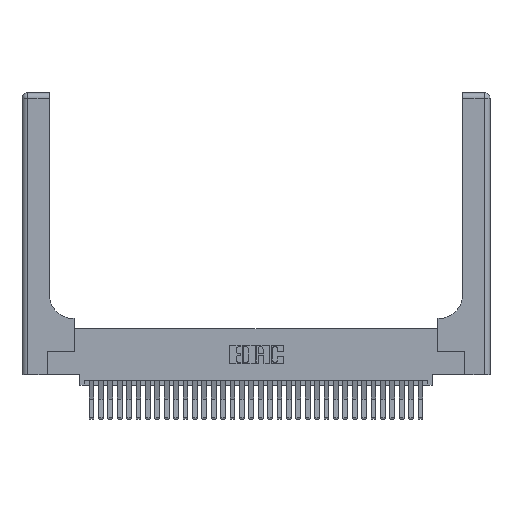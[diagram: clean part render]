
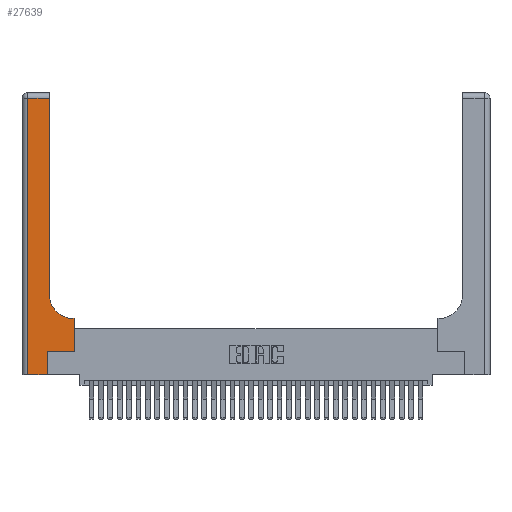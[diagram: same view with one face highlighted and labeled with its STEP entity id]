
A CAD part, top view. The second image highlights one B-rep face of the part: STEP entity #27639.
In plain terms, the highlighted planar face has unit normal (0, 0, 1).
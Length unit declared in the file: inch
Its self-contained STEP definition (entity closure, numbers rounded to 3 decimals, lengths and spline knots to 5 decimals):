
#248 = LINE ( 'NONE', #31415, #19056 ) ;
#401 = EDGE_CURVE ( 'NONE', #17808, #10308, #19400, .T. ) ;
#1413 = VECTOR ( 'NONE', #18477, 39.37008 ) ;
#2298 = LINE ( 'NONE', #22350, #6890 ) ;
#3206 = VERTEX_POINT ( 'NONE', #16425 ) ;
#4150 = DIRECTION ( 'NONE',  ( 0., 1., 0. ) ) ;
#4469 = VECTOR ( 'NONE', #4766, 39.37008 ) ;
#4766 = DIRECTION ( 'NONE',  ( 0., 1., 0. ) ) ;
#5097 = VECTOR ( 'NONE', #6831, 39.37008 ) ;
#5156 = ORIENTED_EDGE ( 'NONE', *, *, #25238, .T. ) ;
#5414 = VERTEX_POINT ( 'NONE', #21873 ) ;
#5603 = LINE ( 'NONE', #12888, #7721 ) ;
#5918 = CARTESIAN_POINT ( 'NONE',  ( 0.2915, 0.85, 0.37 ) ) ;
#6214 = LINE ( 'NONE', #19647, #27952 ) ;
#6332 = DIRECTION ( 'NONE',  ( 0., 0., -1. ) ) ;
#6691 = CARTESIAN_POINT ( 'NONE',  ( 0.269, 0.25, 0.37 ) ) ;
#6831 = DIRECTION ( 'NONE',  ( -1., 0., 0. ) ) ;
#6890 = VECTOR ( 'NONE', #9086, 39.37008 ) ;
#7117 = VERTEX_POINT ( 'NONE', #6691 ) ;
#7645 = CARTESIAN_POINT ( 'NONE',  ( 0.5585, 0.6, 0.37 ) ) ;
#7721 = VECTOR ( 'NONE', #34132, 39.37008 ) ;
#9060 = EDGE_CURVE ( 'NONE', #33289, #17808, #2298, .T. ) ;
#9086 = DIRECTION ( 'NONE',  ( -1., 0., 0. ) ) ;
#9418 = ORIENTED_EDGE ( 'NONE', *, *, #27896, .T. ) ;
#10242 = CARTESIAN_POINT ( 'NONE',  ( 0.269, 0., 0.37 ) ) ;
#10308 = VERTEX_POINT ( 'NONE', #5918 ) ;
#10478 = CARTESIAN_POINT ( 'NONE',  ( 0., 0., 0.37 ) ) ;
#11125 = EDGE_CURVE ( 'NONE', #34152, #5414, #20117, .T. ) ;
#11598 = VECTOR ( 'NONE', #18620, 39.37008 ) ;
#12888 = CARTESIAN_POINT ( 'NONE',  ( 0.269, 0.25, 0.37 ) ) ;
#13156 = FACE_OUTER_BOUND ( 'NONE', #20005, .T. ) ;
#13766 = ORIENTED_EDGE ( 'NONE', *, *, #9060, .T. ) ;
#14985 = CARTESIAN_POINT ( 'NONE',  ( 0., 2.94, 0.37 ) ) ;
#15818 = CARTESIAN_POINT ( 'NONE',  ( 0.06, 0., 0.37 ) ) ;
#16425 = CARTESIAN_POINT ( 'NONE',  ( 0.5585, 0.25, 0.37 ) ) ;
#16432 = LINE ( 'NONE', #10242, #1413 ) ;
#16770 = CARTESIAN_POINT ( 'NONE',  ( 0.2915, 2.94, 0.37 ) ) ;
#17087 = CARTESIAN_POINT ( 'NONE',  ( 0., 3., 0.37 ) ) ;
#17568 = ORIENTED_EDGE ( 'NONE', *, *, #11125, .T. ) ;
#17589 = ORIENTED_EDGE ( 'NONE', *, *, #27932, .T. ) ;
#17808 = VERTEX_POINT ( 'NONE', #27889 ) ;
#18477 = DIRECTION ( 'NONE',  ( 0., 1., 0. ) ) ;
#18620 = DIRECTION ( 'NONE',  ( 1., 0., 0. ) ) ;
#18775 = ORIENTED_EDGE ( 'NONE', *, *, #401, .T. ) ;
#19056 = VECTOR ( 'NONE', #20577, 39.37008 ) ;
#19400 = CIRCLE ( 'NONE', #32054, 0.25 ) ;
#19488 = EDGE_CURVE ( 'NONE', #10308, #34152, #24003, .T. ) ;
#19647 = CARTESIAN_POINT ( 'NONE',  ( 0.5585, 0.25, 0.37 ) ) ;
#19704 = DIRECTION ( 'NONE',  ( 1., 0., 0. ) ) ;
#20005 = EDGE_LOOP ( 'NONE', ( #26227, #17568, #32845, #5156, #17589, #9418, #26740, #13766, #18775 ) ) ;
#20117 = LINE ( 'NONE', #14985, #5097 ) ;
#20577 = DIRECTION ( 'NONE',  ( 0., -1., 0. ) ) ;
#20743 = CARTESIAN_POINT ( 'NONE',  ( 0.2915, 3., 0.37 ) ) ;
#21873 = CARTESIAN_POINT ( 'NONE',  ( 0.06, 2.94, 0.37 ) ) ;
#22350 = CARTESIAN_POINT ( 'NONE',  ( 0.2915, 0.6, 0.37 ) ) ;
#22403 = CARTESIAN_POINT ( 'NONE',  ( 0.269, 0., 0.37 ) ) ;
#24003 = LINE ( 'NONE', #20743, #4469 ) ;
#25238 = EDGE_CURVE ( 'NONE', #29356, #30437, #27428, .T. ) ;
#25849 = EDGE_CURVE ( 'NONE', #5414, #29356, #248, .T. ) ;
#26227 = ORIENTED_EDGE ( 'NONE', *, *, #19488, .T. ) ;
#26740 = ORIENTED_EDGE ( 'NONE', *, *, #31807, .T. ) ;
#26752 = AXIS2_PLACEMENT_3D ( 'NONE', #17087, #6332, #30371 ) ;
#27428 = LINE ( 'NONE', #10478, #11598 ) ;
#27639 = ADVANCED_FACE ( 'NONE', ( #13156 ), #33104, .F. ) ;
#27865 = DIRECTION ( 'NONE',  ( 0., 0., -1. ) ) ;
#27889 = CARTESIAN_POINT ( 'NONE',  ( 0.5415, 0.6, 0.37 ) ) ;
#27896 = EDGE_CURVE ( 'NONE', #7117, #3206, #5603, .T. ) ;
#27932 = EDGE_CURVE ( 'NONE', #30437, #7117, #16432, .T. ) ;
#27952 = VECTOR ( 'NONE', #4150, 39.37008 ) ;
#29356 = VERTEX_POINT ( 'NONE', #15818 ) ;
#30371 = DIRECTION ( 'NONE',  ( -1., 0., 0. ) ) ;
#30437 = VERTEX_POINT ( 'NONE', #22403 ) ;
#31415 = CARTESIAN_POINT ( 'NONE',  ( 0.06, 3., 0.37 ) ) ;
#31807 = EDGE_CURVE ( 'NONE', #3206, #33289, #6214, .T. ) ;
#32054 = AXIS2_PLACEMENT_3D ( 'NONE', #33169, #27865, #19704 ) ;
#32845 = ORIENTED_EDGE ( 'NONE', *, *, #25849, .T. ) ;
#33104 = PLANE ( 'NONE',  #26752 ) ;
#33169 = CARTESIAN_POINT ( 'NONE',  ( 0.5415, 0.85, 0.37 ) ) ;
#33289 = VERTEX_POINT ( 'NONE', #7645 ) ;
#34132 = DIRECTION ( 'NONE',  ( 1., 0., 0. ) ) ;
#34152 = VERTEX_POINT ( 'NONE', #16770 ) ;
